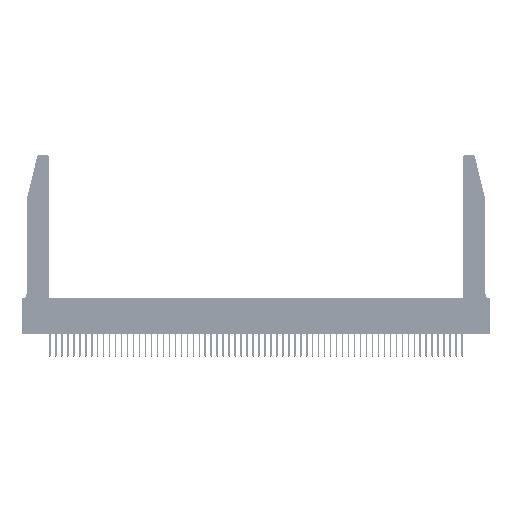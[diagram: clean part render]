
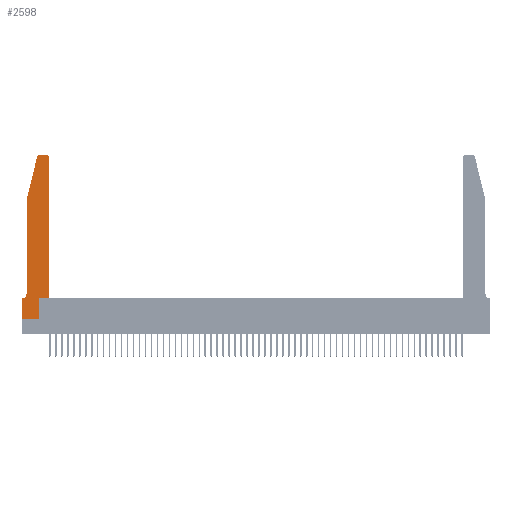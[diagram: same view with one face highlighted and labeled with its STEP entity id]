
A CAD part, top view. The second image highlights one B-rep face of the part: STEP entity #2598.
In plain terms, the highlighted planar face has unit normal (0, 0, 1).
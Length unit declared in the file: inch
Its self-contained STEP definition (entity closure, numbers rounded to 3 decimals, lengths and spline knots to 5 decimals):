
#287 = ORIENTED_EDGE ( 'NONE', *, *, #51529, .T. ) ;
#1029 = CIRCLE ( 'NONE', #4827, 0.03 ) ;
#1793 = VERTEX_POINT ( 'NONE', #12294 ) ;
#2338 = PLANE ( 'NONE',  #45169 ) ;
#2389 = ORIENTED_EDGE ( 'NONE', *, *, #52713, .T. ) ;
#2598 = ADVANCED_FACE ( 'NONE', ( #32750 ), #2338, .T. ) ;
#3162 = EDGE_CURVE ( 'NONE', #17711, #14920, #47630, .T. ) ;
#3259 = DIRECTION ( 'NONE',  ( 0., 0., 1. ) ) ;
#3640 = VECTOR ( 'NONE', #36469, 39.37008 ) ;
#4259 = CARTESIAN_POINT ( 'NONE',  ( 0.0755, 2., 0.37 ) ) ;
#4820 = DIRECTION ( 'NONE',  ( -0.239, -0.971, 0. ) ) ;
#4827 = AXIS2_PLACEMENT_3D ( 'NONE', #42675, #16781, #9217 ) ;
#5686 = CARTESIAN_POINT ( 'NONE',  ( 0.0055, 0.35, 0.37 ) ) ;
#5901 = CARTESIAN_POINT ( 'NONE',  ( 0.0755, 0.35, 0.37 ) ) ;
#7378 = CARTESIAN_POINT ( 'NONE',  ( 0.0055, 0.42, 0.37 ) ) ;
#9217 = DIRECTION ( 'NONE',  ( 1., 0., 0. ) ) ;
#9807 = DIRECTION ( 'NONE',  ( 0., -1., 0. ) ) ;
#10444 = VERTEX_POINT ( 'NONE', #29074 ) ;
#11346 = DIRECTION ( 'NONE',  ( -1., 0., 0. ) ) ;
#11416 = EDGE_CURVE ( 'NONE', #27778, #32089, #26430, .T. ) ;
#12294 = CARTESIAN_POINT ( 'NONE',  ( 0.0755, 0.42, 0.37 ) ) ;
#12407 = LINE ( 'NONE', #5901, #3640 ) ;
#13358 = VECTOR ( 'NONE', #20545, 39.37008 ) ;
#13478 = CARTESIAN_POINT ( 'NONE',  ( 0.4505, 0.35, 0.37 ) ) ;
#14196 = CARTESIAN_POINT ( 'NONE',  ( 0.4505, 0.35, 0.37 ) ) ;
#14296 = VERTEX_POINT ( 'NONE', #39867 ) ;
#14920 = VERTEX_POINT ( 'NONE', #39607 ) ;
#15820 = EDGE_LOOP ( 'NONE', ( #22155, #33870, #19352, #54540, #26749, #19121, #2389, #287, #18315, #45927, #23823, #38915 ) ) ;
#16125 = VERTEX_POINT ( 'NONE', #5686 ) ;
#16781 = DIRECTION ( 'NONE',  ( 0., 0., 1. ) ) ;
#16856 = AXIS2_PLACEMENT_3D ( 'NONE', #30512, #38687, #47380 ) ;
#16906 = DIRECTION ( 'NONE',  ( 0., -1., 0. ) ) ;
#17711 = VERTEX_POINT ( 'NONE', #40370 ) ;
#18315 = ORIENTED_EDGE ( 'NONE', *, *, #3162, .T. ) ;
#18494 = CARTESIAN_POINT ( 'NONE',  ( 0., 0., 0.37 ) ) ;
#18634 = DIRECTION ( 'NONE',  ( 1., 0., 0. ) ) ;
#19121 = ORIENTED_EDGE ( 'NONE', *, *, #54071, .T. ) ;
#19141 = VERTEX_POINT ( 'NONE', #38135 ) ;
#19149 = VERTEX_POINT ( 'NONE', #46845 ) ;
#19225 = LINE ( 'NONE', #42259, #52343 ) ;
#19352 = ORIENTED_EDGE ( 'NONE', *, *, #43246, .T. ) ;
#19975 = DIRECTION ( 'NONE',  ( -1., 0., 0. ) ) ;
#20478 = DIRECTION ( 'NONE',  ( 1., 0., 0. ) ) ;
#20545 = DIRECTION ( 'NONE',  ( 1., 0., 0. ) ) ;
#20604 = EDGE_CURVE ( 'NONE', #14920, #51995, #34974, .T. ) ;
#20928 = CARTESIAN_POINT ( 'NONE',  ( 0.4505, 0.35, 0.37 ) ) ;
#22080 = LINE ( 'NONE', #18494, #48434 ) ;
#22155 = ORIENTED_EDGE ( 'NONE', *, *, #34876, .T. ) ;
#22553 = VECTOR ( 'NONE', #16906, 39.37008 ) ;
#22888 = EDGE_CURVE ( 'NONE', #14296, #1793, #42182, .T. ) ;
#23102 = VERTEX_POINT ( 'NONE', #32146 ) ;
#23823 = ORIENTED_EDGE ( 'NONE', *, *, #50057, .T. ) ;
#24555 = DIRECTION ( 'NONE',  ( 0., 1., 0. ) ) ;
#26430 = CIRCLE ( 'NONE', #16856, 0.03 ) ;
#26524 = DIRECTION ( 'NONE',  ( 0., 1., 0. ) ) ;
#26749 = ORIENTED_EDGE ( 'NONE', *, *, #54145, .T. ) ;
#27778 = VERTEX_POINT ( 'NONE', #29391 ) ;
#29074 = CARTESIAN_POINT ( 'NONE',  ( 0.4505, 2.72, 0.37 ) ) ;
#29391 = CARTESIAN_POINT ( 'NONE',  ( 0.284, 2.75, 0.37 ) ) ;
#30512 = CARTESIAN_POINT ( 'NONE',  ( 0.284, 2.72, 0.37 ) ) ;
#32089 = VERTEX_POINT ( 'NONE', #43338 ) ;
#32146 = CARTESIAN_POINT ( 'NONE',  ( 0., 0., 0.37 ) ) ;
#32750 = FACE_OUTER_BOUND ( 'NONE', #15820, .T. ) ;
#33396 = DIRECTION ( 'NONE',  ( 0., 0., -1. ) ) ;
#33870 = ORIENTED_EDGE ( 'NONE', *, *, #11416, .T. ) ;
#34510 = EDGE_CURVE ( 'NONE', #10444, #19141, #1029, .T. ) ;
#34706 = CIRCLE ( 'NONE', #40917, 0.07 ) ;
#34876 = EDGE_CURVE ( 'NONE', #19141, #27778, #19225, .T. ) ;
#34974 = LINE ( 'NONE', #20928, #13358 ) ;
#36469 = DIRECTION ( 'NONE',  ( -1., 0., 0. ) ) ;
#36774 = LINE ( 'NONE', #49239, #41513 ) ;
#38135 = CARTESIAN_POINT ( 'NONE',  ( 0.4205, 2.75, 0.37 ) ) ;
#38167 = CARTESIAN_POINT ( 'NONE',  ( 0.2865, 0.35, 0.37 ) ) ;
#38687 = DIRECTION ( 'NONE',  ( 0., 0., 1. ) ) ;
#38915 = ORIENTED_EDGE ( 'NONE', *, *, #34510, .T. ) ;
#38987 = LINE ( 'NONE', #13478, #49153 ) ;
#39182 = CARTESIAN_POINT ( 'NONE',  ( 0.0755, 2., 0.37 ) ) ;
#39607 = CARTESIAN_POINT ( 'NONE',  ( 0.2865, 0.35, 0.37 ) ) ;
#39867 = CARTESIAN_POINT ( 'NONE',  ( 0.0755, 2., 0.37 ) ) ;
#40370 = CARTESIAN_POINT ( 'NONE',  ( 0.2865, 0., 0.37 ) ) ;
#40917 = AXIS2_PLACEMENT_3D ( 'NONE', #7378, #33396, #11346 ) ;
#41513 = VECTOR ( 'NONE', #18634, 39.37008 ) ;
#42182 = LINE ( 'NONE', #4259, #22553 ) ;
#42259 = CARTESIAN_POINT ( 'NONE',  ( 0.2605, 2.75, 0.37 ) ) ;
#42675 = CARTESIAN_POINT ( 'NONE',  ( 0.4205, 2.72, 0.37 ) ) ;
#42877 = LINE ( 'NONE', #39182, #48303 ) ;
#43246 = EDGE_CURVE ( 'NONE', #32089, #14296, #42877, .T. ) ;
#43338 = CARTESIAN_POINT ( 'NONE',  ( 0.25487, 2.72718, 0.37 ) ) ;
#45169 = AXIS2_PLACEMENT_3D ( 'NONE', #50500, #3259, #20478 ) ;
#45927 = ORIENTED_EDGE ( 'NONE', *, *, #20604, .T. ) ;
#46845 = CARTESIAN_POINT ( 'NONE',  ( 0., 0.35, 0.37 ) ) ;
#47380 = DIRECTION ( 'NONE',  ( 1., 0., 0. ) ) ;
#47630 = LINE ( 'NONE', #38167, #55739 ) ;
#48303 = VECTOR ( 'NONE', #4820, 39.37008 ) ;
#48434 = VECTOR ( 'NONE', #9807, 39.37008 ) ;
#49153 = VECTOR ( 'NONE', #26524, 39.37008 ) ;
#49239 = CARTESIAN_POINT ( 'NONE',  ( 0., 0., 0.37 ) ) ;
#50057 = EDGE_CURVE ( 'NONE', #51995, #10444, #38987, .T. ) ;
#50500 = CARTESIAN_POINT ( 'NONE',  ( 0., 0.35, 0.37 ) ) ;
#51529 = EDGE_CURVE ( 'NONE', #23102, #17711, #36774, .T. ) ;
#51995 = VERTEX_POINT ( 'NONE', #14196 ) ;
#52343 = VECTOR ( 'NONE', #19975, 39.37008 ) ;
#52713 = EDGE_CURVE ( 'NONE', #19149, #23102, #22080, .T. ) ;
#54071 = EDGE_CURVE ( 'NONE', #16125, #19149, #12407, .T. ) ;
#54145 = EDGE_CURVE ( 'NONE', #1793, #16125, #34706, .T. ) ;
#54540 = ORIENTED_EDGE ( 'NONE', *, *, #22888, .T. ) ;
#55739 = VECTOR ( 'NONE', #24555, 39.37008 ) ;
